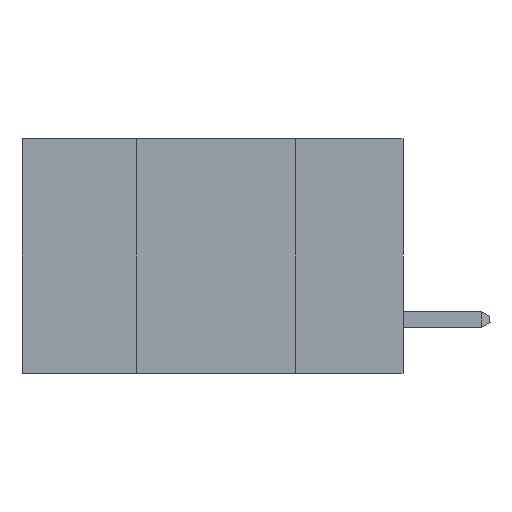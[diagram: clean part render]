
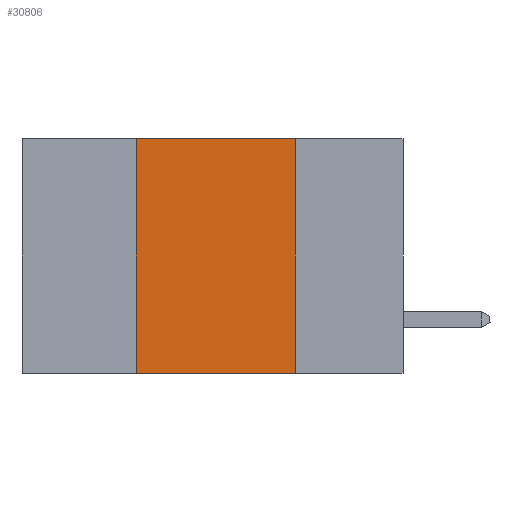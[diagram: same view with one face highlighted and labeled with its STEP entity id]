
A CAD part, left-side view. The second image highlights one B-rep face of the part: STEP entity #30806.
In plain terms, the highlighted planar face has unit normal (-1, 0, 0).
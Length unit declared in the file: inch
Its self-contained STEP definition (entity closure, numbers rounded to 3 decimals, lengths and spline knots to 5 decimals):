
#2059 = CARTESIAN_POINT ( 'NONE',  ( 0., 0.17, 0. ) ) ;
#2394 = DIRECTION ( 'NONE',  ( 0., 0., 1. ) ) ;
#2496 = LINE ( 'NONE', #38668, #28485 ) ;
#3921 = AXIS2_PLACEMENT_3D ( 'NONE', #14289, #10209, #19146 ) ;
#5594 = ORIENTED_EDGE ( 'NONE', *, *, #17024, .F. ) ;
#5757 = VECTOR ( 'NONE', #5763, 39.37008 ) ;
#5763 = DIRECTION ( 'NONE',  ( 0., -1., 0. ) ) ;
#5869 = VERTEX_POINT ( 'NONE', #37836 ) ;
#6723 = VECTOR ( 'NONE', #25881, 39.37008 ) ;
#7383 = LINE ( 'NONE', #37727, #36326 ) ;
#8335 = VERTEX_POINT ( 'NONE', #36460 ) ;
#10209 = DIRECTION ( 'NONE',  ( 1., 0., 0. ) ) ;
#12382 = VERTEX_POINT ( 'NONE', #34428 ) ;
#14289 = CARTESIAN_POINT ( 'NONE',  ( 0., 0.6, 0. ) ) ;
#15676 = LINE ( 'NONE', #26277, #5757 ) ;
#17024 = EDGE_CURVE ( 'NONE', #28903, #12382, #26159, .T. ) ;
#18493 = FACE_OUTER_BOUND ( 'NONE', #21112, .T. ) ;
#19146 = DIRECTION ( 'NONE',  ( 0., 0., -1. ) ) ;
#19601 = DIRECTION ( 'NONE',  ( 0., -1., 0. ) ) ;
#20142 = EDGE_CURVE ( 'NONE', #8335, #12382, #7383, .T. ) ;
#21112 = EDGE_LOOP ( 'NONE', ( #5594, #36590, #35986, #38456 ) ) ;
#25060 = EDGE_CURVE ( 'NONE', #8335, #5869, #2496, .T. ) ;
#25881 = DIRECTION ( 'NONE',  ( 0., 0., -1. ) ) ;
#26159 = LINE ( 'NONE', #2059, #6723 ) ;
#26277 = CARTESIAN_POINT ( 'NONE',  ( 0., 0.6, 0. ) ) ;
#26840 = PLANE ( 'NONE',  #3921 ) ;
#28485 = VECTOR ( 'NONE', #2394, 39.37008 ) ;
#28903 = VERTEX_POINT ( 'NONE', #35864 ) ;
#30806 = ADVANCED_FACE ( 'NONE', ( #18493 ), #26840, .F. ) ;
#34428 = CARTESIAN_POINT ( 'NONE',  ( 0., 0.17, -0.37 ) ) ;
#35864 = CARTESIAN_POINT ( 'NONE',  ( 0., 0.17, 0. ) ) ;
#35986 = ORIENTED_EDGE ( 'NONE', *, *, #25060, .F. ) ;
#36326 = VECTOR ( 'NONE', #19601, 39.37008 ) ;
#36460 = CARTESIAN_POINT ( 'NONE',  ( 0., 0.42, -0.37 ) ) ;
#36590 = ORIENTED_EDGE ( 'NONE', *, *, #37538, .F. ) ;
#37538 = EDGE_CURVE ( 'NONE', #5869, #28903, #15676, .T. ) ;
#37727 = CARTESIAN_POINT ( 'NONE',  ( 0., 0.6, -0.37 ) ) ;
#37836 = CARTESIAN_POINT ( 'NONE',  ( 0., 0.42, 0. ) ) ;
#38456 = ORIENTED_EDGE ( 'NONE', *, *, #20142, .T. ) ;
#38668 = CARTESIAN_POINT ( 'NONE',  ( 0., 0.42, 0. ) ) ;
